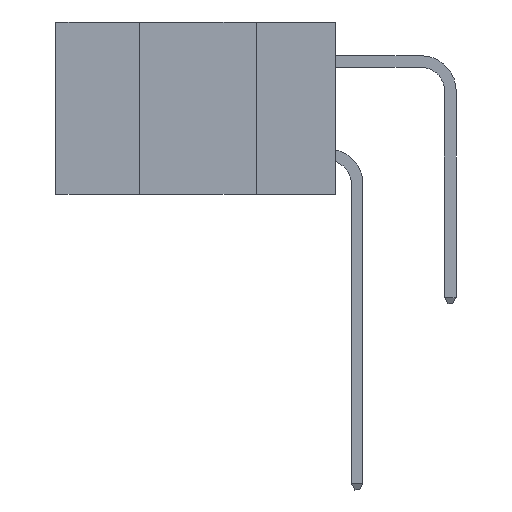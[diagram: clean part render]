
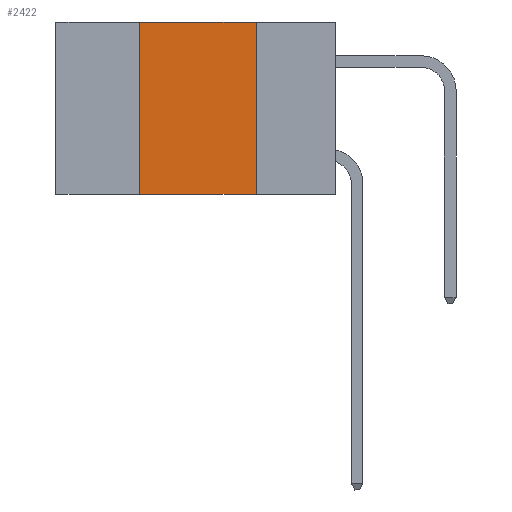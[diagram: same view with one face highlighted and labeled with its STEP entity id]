
A CAD part, left-side view. The second image highlights one B-rep face of the part: STEP entity #2422.
In plain terms, the highlighted planar face has unit normal (-1, 0, 0).
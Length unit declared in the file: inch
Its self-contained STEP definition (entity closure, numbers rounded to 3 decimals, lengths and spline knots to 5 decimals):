
#1093 = LINE ( 'NONE', #1214, #9471 ) ;
#1151 = LINE ( 'NONE', #1343, #3775 ) ;
#1214 = CARTESIAN_POINT ( 'NONE',  ( 0., 0.6, -0.37 ) ) ;
#1343 = CARTESIAN_POINT ( 'NONE',  ( 0., 0.42, 0. ) ) ;
#1351 = CARTESIAN_POINT ( 'NONE',  ( 0., 0.17, 0. ) ) ;
#1374 = DIRECTION ( 'NONE',  ( 0., 0., 1. ) ) ;
#1717 = EDGE_CURVE ( 'NONE', #11290, #10183, #1151, .T. ) ;
#2361 = DIRECTION ( 'NONE',  ( 0., -1., 0. ) ) ;
#2422 = ADVANCED_FACE ( 'NONE', ( #12522 ), #3497, .F. ) ;
#3200 = CARTESIAN_POINT ( 'NONE',  ( 0., 0.42, 0. ) ) ;
#3497 = PLANE ( 'NONE',  #8865 ) ;
#3644 = VERTEX_POINT ( 'NONE', #5623 ) ;
#3693 = VERTEX_POINT ( 'NONE', #10004 ) ;
#3775 = VECTOR ( 'NONE', #1374, 39.37008 ) ;
#3977 = DIRECTION ( 'NONE',  ( 0., -1., 0. ) ) ;
#4586 = DIRECTION ( 'NONE',  ( 1., 0., 0. ) ) ;
#5623 = CARTESIAN_POINT ( 'NONE',  ( 0., 0.17, 0. ) ) ;
#7253 = ORIENTED_EDGE ( 'NONE', *, *, #10578, .F. ) ;
#7506 = LINE ( 'NONE', #1351, #12308 ) ;
#7650 = EDGE_CURVE ( 'NONE', #11290, #3693, #1093, .T. ) ;
#7963 = DIRECTION ( 'NONE',  ( 0., 0., -1. ) ) ;
#8437 = VECTOR ( 'NONE', #3977, 39.37008 ) ;
#8865 = AXIS2_PLACEMENT_3D ( 'NONE', #10967, #4586, #11966 ) ;
#9471 = VECTOR ( 'NONE', #2361, 39.37008 ) ;
#10004 = CARTESIAN_POINT ( 'NONE',  ( 0., 0.17, -0.37 ) ) ;
#10183 = VERTEX_POINT ( 'NONE', #3200 ) ;
#10408 = CARTESIAN_POINT ( 'NONE',  ( 0., 0.6, 0. ) ) ;
#10578 = EDGE_CURVE ( 'NONE', #10183, #3644, #13512, .T. ) ;
#10680 = ORIENTED_EDGE ( 'NONE', *, *, #7650, .T. ) ;
#10967 = CARTESIAN_POINT ( 'NONE',  ( 0., 0.6, 0. ) ) ;
#11290 = VERTEX_POINT ( 'NONE', #12516 ) ;
#11449 = ORIENTED_EDGE ( 'NONE', *, *, #13376, .F. ) ;
#11561 = EDGE_LOOP ( 'NONE', ( #11449, #7253, #13038, #10680 ) ) ;
#11966 = DIRECTION ( 'NONE',  ( 0., 0., -1. ) ) ;
#12308 = VECTOR ( 'NONE', #7963, 39.37008 ) ;
#12516 = CARTESIAN_POINT ( 'NONE',  ( 0., 0.42, -0.37 ) ) ;
#12522 = FACE_OUTER_BOUND ( 'NONE', #11561, .T. ) ;
#13038 = ORIENTED_EDGE ( 'NONE', *, *, #1717, .F. ) ;
#13376 = EDGE_CURVE ( 'NONE', #3644, #3693, #7506, .T. ) ;
#13512 = LINE ( 'NONE', #10408, #8437 ) ;
